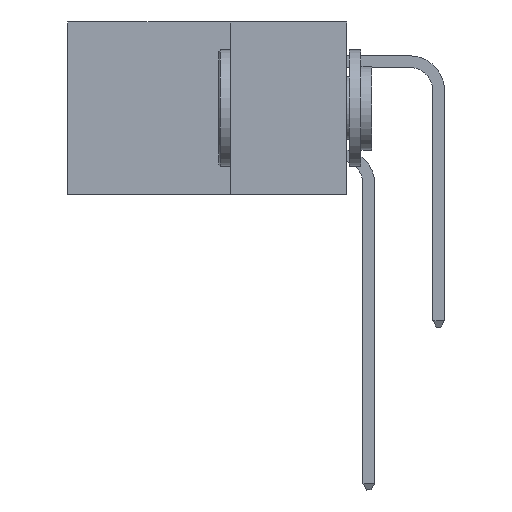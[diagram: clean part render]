
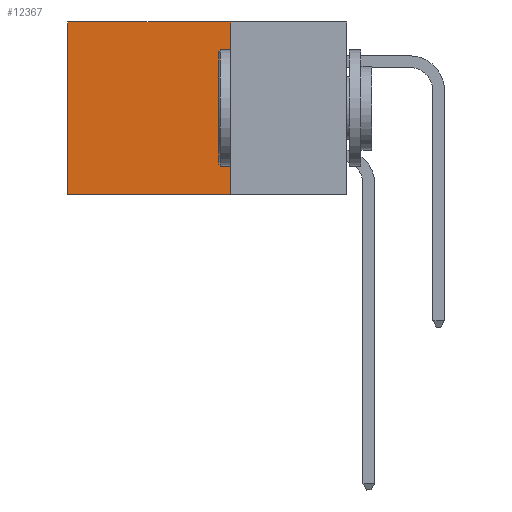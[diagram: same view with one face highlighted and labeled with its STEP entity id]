
A CAD part, left-side view. The second image highlights one B-rep face of the part: STEP entity #12367.
In plain terms, the highlighted planar face has unit normal (-1, 0, 0).
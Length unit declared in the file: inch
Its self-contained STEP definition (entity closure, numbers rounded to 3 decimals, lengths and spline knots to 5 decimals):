
#67 = CARTESIAN_POINT ( 'NONE',  ( 0.2875, 0.25, 0. ) ) ;
#163 = ORIENTED_EDGE ( 'NONE', *, *, #33558, .F. ) ;
#937 = VECTOR ( 'NONE', #8116, 39.37008 ) ;
#1717 = VECTOR ( 'NONE', #12136, 39.37008 ) ;
#3467 = LINE ( 'NONE', #25571, #30512 ) ;
#3660 = CARTESIAN_POINT ( 'NONE',  ( 0.2875, 0.25, 0. ) ) ;
#3874 = CARTESIAN_POINT ( 'NONE',  ( 0.2875, 0.6, 0. ) ) ;
#4959 = VECTOR ( 'NONE', #15135, 39.37008 ) ;
#5209 = VERTEX_POINT ( 'NONE', #6465 ) ;
#6127 = CARTESIAN_POINT ( 'NONE',  ( 0.2875, 0.6, -0.37 ) ) ;
#6188 = DIRECTION ( 'NONE',  ( 1., 0., 0. ) ) ;
#6465 = CARTESIAN_POINT ( 'NONE',  ( 0.2875, 0.25, -0.37 ) ) ;
#8116 = DIRECTION ( 'NONE',  ( 0., 1., 0. ) ) ;
#8678 = ORIENTED_EDGE ( 'NONE', *, *, #33104, .T. ) ;
#8684 = DIRECTION ( 'NONE',  ( 0., 1., 0. ) ) ;
#9142 = PLANE ( 'NONE',  #20836 ) ;
#12136 = DIRECTION ( 'NONE',  ( 0., 0., -1. ) ) ;
#12367 = ADVANCED_FACE ( 'NONE', ( #33013 ), #9142, .F. ) ;
#14639 = VERTEX_POINT ( 'NONE', #3660 ) ;
#15135 = DIRECTION ( 'NONE',  ( 0., 0., -1. ) ) ;
#16385 = LINE ( 'NONE', #67, #937 ) ;
#17335 = VERTEX_POINT ( 'NONE', #3874 ) ;
#17454 = EDGE_CURVE ( 'NONE', #14639, #5209, #25244, .T. ) ;
#17671 = DIRECTION ( 'NONE',  ( 0., 0., -1. ) ) ;
#18211 = EDGE_LOOP ( 'NONE', ( #8678, #163, #30905, #20500 ) ) ;
#18897 = EDGE_CURVE ( 'NONE', #14639, #17335, #16385, .T. ) ;
#20500 = ORIENTED_EDGE ( 'NONE', *, *, #18897, .T. ) ;
#20519 = CARTESIAN_POINT ( 'NONE',  ( 0.2875, 0.6, 0. ) ) ;
#20836 = AXIS2_PLACEMENT_3D ( 'NONE', #28989, #6188, #17671 ) ;
#22506 = LINE ( 'NONE', #20519, #1717 ) ;
#22533 = VERTEX_POINT ( 'NONE', #6127 ) ;
#25244 = LINE ( 'NONE', #31038, #4959 ) ;
#25571 = CARTESIAN_POINT ( 'NONE',  ( 0.2875, 0.25, -0.37 ) ) ;
#28989 = CARTESIAN_POINT ( 'NONE',  ( 0.2875, 0.25, 0. ) ) ;
#30512 = VECTOR ( 'NONE', #8684, 39.37008 ) ;
#30905 = ORIENTED_EDGE ( 'NONE', *, *, #17454, .F. ) ;
#31038 = CARTESIAN_POINT ( 'NONE',  ( 0.2875, 0.25, 0. ) ) ;
#33013 = FACE_OUTER_BOUND ( 'NONE', #18211, .T. ) ;
#33104 = EDGE_CURVE ( 'NONE', #17335, #22533, #22506, .T. ) ;
#33558 = EDGE_CURVE ( 'NONE', #5209, #22533, #3467, .T. ) ;
